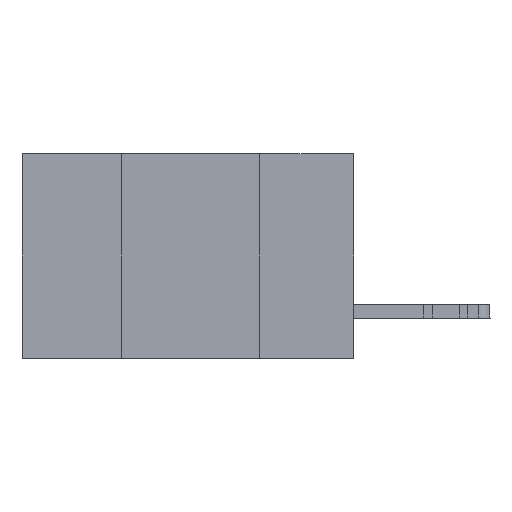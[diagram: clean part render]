
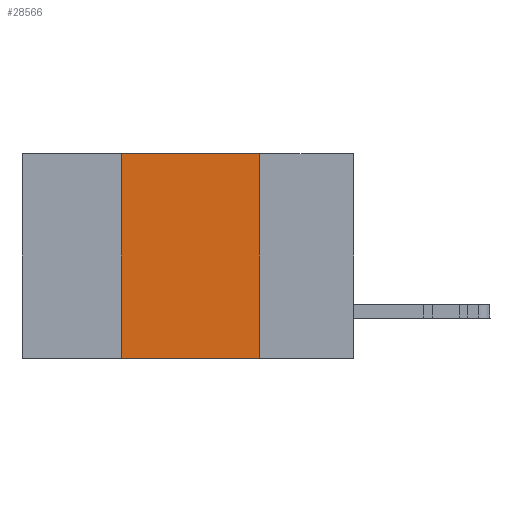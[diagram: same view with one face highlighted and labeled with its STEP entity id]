
A CAD part, left-side view. The second image highlights one B-rep face of the part: STEP entity #28566.
In plain terms, the highlighted planar face has unit normal (-1, 0, 0).
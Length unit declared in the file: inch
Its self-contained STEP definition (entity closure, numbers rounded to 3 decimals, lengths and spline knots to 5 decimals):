
#152 = DIRECTION ( 'NONE',  ( 0., 0., 1. ) ) ;
#182 = ORIENTED_EDGE ( 'NONE', *, *, #28254, .F. ) ;
#1839 = VERTEX_POINT ( 'NONE', #33445 ) ;
#5575 = EDGE_CURVE ( 'NONE', #34240, #14670, #14428, .T. ) ;
#6907 = CARTESIAN_POINT ( 'NONE',  ( 0., 0.6, 0. ) ) ;
#7210 = VECTOR ( 'NONE', #33236, 39.37008 ) ;
#7330 = EDGE_LOOP ( 'NONE', ( #182, #32952, #18884, #18426 ) ) ;
#7864 = DIRECTION ( 'NONE',  ( 0., -1., 0. ) ) ;
#12528 = DIRECTION ( 'NONE',  ( 1., 0., 0. ) ) ;
#12616 = CARTESIAN_POINT ( 'NONE',  ( 0., 0.42, -0.37 ) ) ;
#13931 = CARTESIAN_POINT ( 'NONE',  ( 0., 0.17, 0. ) ) ;
#14428 = LINE ( 'NONE', #6907, #16411 ) ;
#14517 = EDGE_CURVE ( 'NONE', #31380, #1839, #14722, .T. ) ;
#14670 = VERTEX_POINT ( 'NONE', #13931 ) ;
#14722 = LINE ( 'NONE', #33057, #36420 ) ;
#15680 = AXIS2_PLACEMENT_3D ( 'NONE', #28494, #12528, #31677 ) ;
#16411 = VECTOR ( 'NONE', #7864, 39.37008 ) ;
#18426 = ORIENTED_EDGE ( 'NONE', *, *, #14517, .T. ) ;
#18884 = ORIENTED_EDGE ( 'NONE', *, *, #40009, .F. ) ;
#20628 = DIRECTION ( 'NONE',  ( 0., -1., 0. ) ) ;
#22037 = CARTESIAN_POINT ( 'NONE',  ( 0., 0.42, 0. ) ) ;
#22460 = VECTOR ( 'NONE', #152, 39.37008 ) ;
#28254 = EDGE_CURVE ( 'NONE', #14670, #1839, #40392, .T. ) ;
#28494 = CARTESIAN_POINT ( 'NONE',  ( 0., 0.6, 0. ) ) ;
#28566 = ADVANCED_FACE ( 'NONE', ( #31961 ), #37880, .F. ) ;
#31167 = CARTESIAN_POINT ( 'NONE',  ( 0., 0.42, 0. ) ) ;
#31380 = VERTEX_POINT ( 'NONE', #12616 ) ;
#31677 = DIRECTION ( 'NONE',  ( 0., 0., -1. ) ) ;
#31961 = FACE_OUTER_BOUND ( 'NONE', #7330, .T. ) ;
#32952 = ORIENTED_EDGE ( 'NONE', *, *, #5575, .F. ) ;
#33057 = CARTESIAN_POINT ( 'NONE',  ( 0., 0.6, -0.37 ) ) ;
#33236 = DIRECTION ( 'NONE',  ( 0., 0., -1. ) ) ;
#33445 = CARTESIAN_POINT ( 'NONE',  ( 0., 0.17, -0.37 ) ) ;
#34240 = VERTEX_POINT ( 'NONE', #31167 ) ;
#35208 = LINE ( 'NONE', #22037, #22460 ) ;
#36420 = VECTOR ( 'NONE', #20628, 39.37008 ) ;
#36795 = CARTESIAN_POINT ( 'NONE',  ( 0., 0.17, 0. ) ) ;
#37880 = PLANE ( 'NONE',  #15680 ) ;
#40009 = EDGE_CURVE ( 'NONE', #31380, #34240, #35208, .T. ) ;
#40392 = LINE ( 'NONE', #36795, #7210 ) ;
